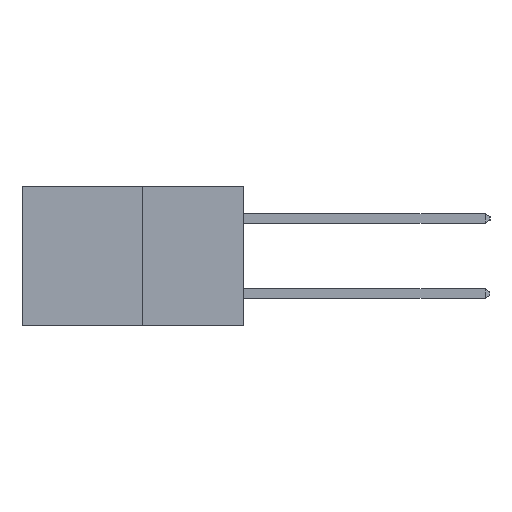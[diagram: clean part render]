
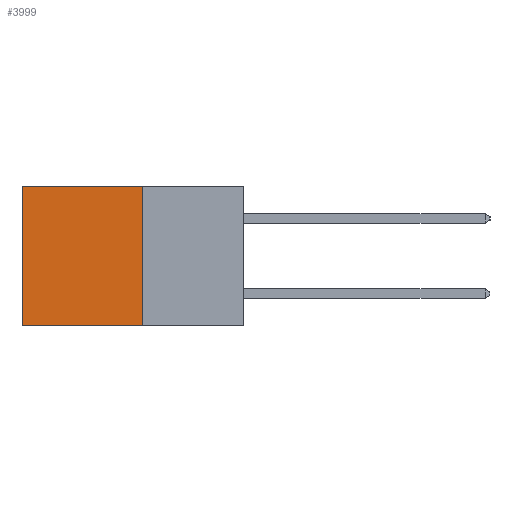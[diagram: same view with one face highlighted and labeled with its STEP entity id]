
A CAD part, left-side view. The second image highlights one B-rep face of the part: STEP entity #3999.
In plain terms, the highlighted planar face has unit normal (-1, 0, 0).
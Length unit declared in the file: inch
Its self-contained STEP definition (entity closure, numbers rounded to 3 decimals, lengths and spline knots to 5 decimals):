
#317 = DIRECTION ( 'NONE',  ( 0., 0., -1. ) ) ;
#434 = VERTEX_POINT ( 'NONE', #3427 ) ;
#568 = CARTESIAN_POINT ( 'NONE',  ( 0.277, 0.59, 0. ) ) ;
#581 = CARTESIAN_POINT ( 'NONE',  ( 0.277, 0.27, -0.37 ) ) ;
#912 = VECTOR ( 'NONE', #8221, 39.37008 ) ;
#928 = FACE_OUTER_BOUND ( 'NONE', #4158, .T. ) ;
#1041 = AXIS2_PLACEMENT_3D ( 'NONE', #1907, #3942, #2488 ) ;
#1140 = EDGE_CURVE ( 'NONE', #4749, #5769, #5900, .T. ) ;
#1234 = VERTEX_POINT ( 'NONE', #5834 ) ;
#1270 = VECTOR ( 'NONE', #317, 39.37008 ) ;
#1656 = ORIENTED_EDGE ( 'NONE', *, *, #6080, .T. ) ;
#1907 = CARTESIAN_POINT ( 'NONE',  ( 0.277, 0.27, -0.37 ) ) ;
#2144 = VECTOR ( 'NONE', #5383, 39.37008 ) ;
#2488 = DIRECTION ( 'NONE',  ( 0., 0., -1. ) ) ;
#2985 = ORIENTED_EDGE ( 'NONE', *, *, #1140, .T. ) ;
#3427 = CARTESIAN_POINT ( 'NONE',  ( 0.277, 0.27, -0.37 ) ) ;
#3726 = CARTESIAN_POINT ( 'NONE',  ( 0.277, 0.27, 0. ) ) ;
#3942 = DIRECTION ( 'NONE',  ( 1., 0., 0. ) ) ;
#3999 = ADVANCED_FACE ( 'NONE', ( #928 ), #6398, .F. ) ;
#4158 = EDGE_LOOP ( 'NONE', ( #2985, #6873, #6923, #1656 ) ) ;
#4298 = CARTESIAN_POINT ( 'NONE',  ( 0.277, 0.59, -0.37 ) ) ;
#4749 = VERTEX_POINT ( 'NONE', #568 ) ;
#4954 = EDGE_CURVE ( 'NONE', #434, #5769, #6029, .T. ) ;
#5383 = DIRECTION ( 'NONE',  ( 0., 1., 0. ) ) ;
#5413 = DIRECTION ( 'NONE',  ( 0., 0., -1. ) ) ;
#5769 = VERTEX_POINT ( 'NONE', #8385 ) ;
#5834 = CARTESIAN_POINT ( 'NONE',  ( 0.277, 0.27, 0. ) ) ;
#5900 = LINE ( 'NONE', #4298, #7410 ) ;
#6029 = LINE ( 'NONE', #6613, #912 ) ;
#6080 = EDGE_CURVE ( 'NONE', #1234, #4749, #7420, .T. ) ;
#6398 = PLANE ( 'NONE',  #1041 ) ;
#6613 = CARTESIAN_POINT ( 'NONE',  ( 0.277, 0.27, -0.37 ) ) ;
#6873 = ORIENTED_EDGE ( 'NONE', *, *, #4954, .F. ) ;
#6923 = ORIENTED_EDGE ( 'NONE', *, *, #7990, .F. ) ;
#7410 = VECTOR ( 'NONE', #5413, 39.37008 ) ;
#7420 = LINE ( 'NONE', #3726, #2144 ) ;
#7990 = EDGE_CURVE ( 'NONE', #1234, #434, #8199, .T. ) ;
#8199 = LINE ( 'NONE', #581, #1270 ) ;
#8221 = DIRECTION ( 'NONE',  ( 0., 1., 0. ) ) ;
#8385 = CARTESIAN_POINT ( 'NONE',  ( 0.277, 0.59, -0.37 ) ) ;
